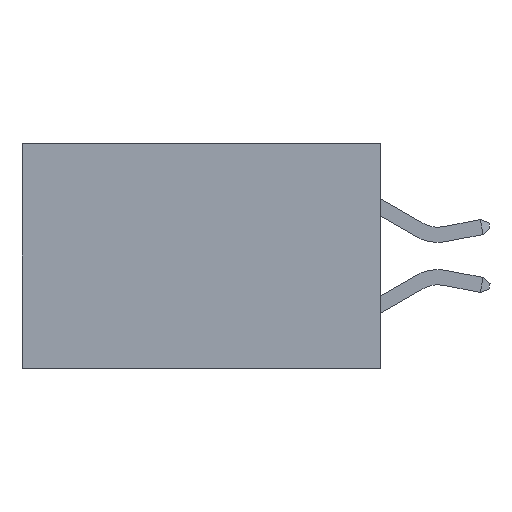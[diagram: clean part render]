
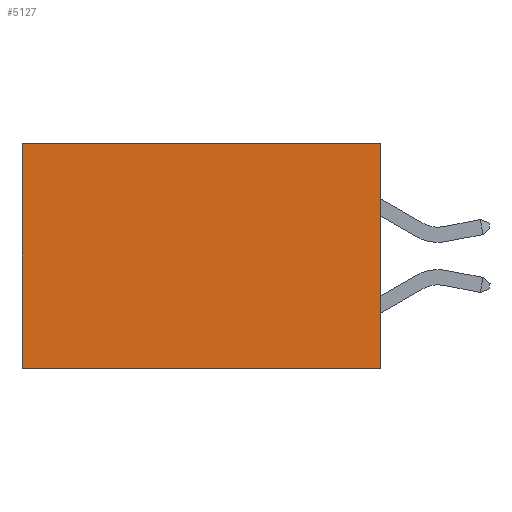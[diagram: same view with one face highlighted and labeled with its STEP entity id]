
A CAD part, left-side view. The second image highlights one B-rep face of the part: STEP entity #5127.
In plain terms, the highlighted planar face has unit normal (-1, 0, 0).
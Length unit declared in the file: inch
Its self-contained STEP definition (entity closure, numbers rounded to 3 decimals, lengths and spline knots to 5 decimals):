
#86 = CARTESIAN_POINT ( 'NONE',  ( 0.277, 0.59, -0.37 ) ) ;
#1975 = VECTOR ( 'NONE', #13735, 39.37008 ) ;
#2057 = VECTOR ( 'NONE', #12138, 39.37008 ) ;
#2641 = CARTESIAN_POINT ( 'NONE',  ( 0.277, 0., -0.37 ) ) ;
#2697 = DIRECTION ( 'NONE',  ( 1., 0., 0. ) ) ;
#3251 = FACE_OUTER_BOUND ( 'NONE', #6950, .T. ) ;
#3413 = LINE ( 'NONE', #5253, #16617 ) ;
#3823 = CARTESIAN_POINT ( 'NONE',  ( 0.277, 0., -0.37 ) ) ;
#4322 = DIRECTION ( 'NONE',  ( 0., 0., -1. ) ) ;
#4506 = CARTESIAN_POINT ( 'NONE',  ( 0.277, 0., -0.37 ) ) ;
#4891 = PLANE ( 'NONE',  #14306 ) ;
#5127 = ADVANCED_FACE ( 'NONE', ( #3251 ), #4891, .F. ) ;
#5253 = CARTESIAN_POINT ( 'NONE',  ( 0.277, 0., -0.37 ) ) ;
#6950 = EDGE_LOOP ( 'NONE', ( #16054, #8222, #9493, #8336 ) ) ;
#7753 = VECTOR ( 'NONE', #10658, 39.37008 ) ;
#8146 = EDGE_CURVE ( 'NONE', #13239, #11355, #11682, .T. ) ;
#8222 = ORIENTED_EDGE ( 'NONE', *, *, #12940, .F. ) ;
#8336 = ORIENTED_EDGE ( 'NONE', *, *, #14643, .T. ) ;
#8605 = LINE ( 'NONE', #4506, #1975 ) ;
#9493 = ORIENTED_EDGE ( 'NONE', *, *, #12369, .F. ) ;
#10575 = DIRECTION ( 'NONE',  ( 0., 1., 0. ) ) ;
#10658 = DIRECTION ( 'NONE',  ( 0., 0., -1. ) ) ;
#11355 = VERTEX_POINT ( 'NONE', #12728 ) ;
#11682 = LINE ( 'NONE', #86, #7753 ) ;
#12138 = DIRECTION ( 'NONE',  ( 0., 1., 0. ) ) ;
#12369 = EDGE_CURVE ( 'NONE', #14615, #15583, #8605, .T. ) ;
#12728 = CARTESIAN_POINT ( 'NONE',  ( 0.277, 0.59, -0.37 ) ) ;
#12940 = EDGE_CURVE ( 'NONE', #15583, #11355, #3413, .T. ) ;
#13239 = VERTEX_POINT ( 'NONE', #15108 ) ;
#13457 = CARTESIAN_POINT ( 'NONE',  ( 0.277, 0., 0. ) ) ;
#13735 = DIRECTION ( 'NONE',  ( 0., 0., -1. ) ) ;
#14306 = AXIS2_PLACEMENT_3D ( 'NONE', #2641, #2697, #4322 ) ;
#14615 = VERTEX_POINT ( 'NONE', #14712 ) ;
#14643 = EDGE_CURVE ( 'NONE', #14615, #13239, #16106, .T. ) ;
#14712 = CARTESIAN_POINT ( 'NONE',  ( 0.277, 0., 0. ) ) ;
#15108 = CARTESIAN_POINT ( 'NONE',  ( 0.277, 0.59, 0. ) ) ;
#15583 = VERTEX_POINT ( 'NONE', #3823 ) ;
#16054 = ORIENTED_EDGE ( 'NONE', *, *, #8146, .T. ) ;
#16106 = LINE ( 'NONE', #13457, #2057 ) ;
#16617 = VECTOR ( 'NONE', #10575, 39.37008 ) ;
